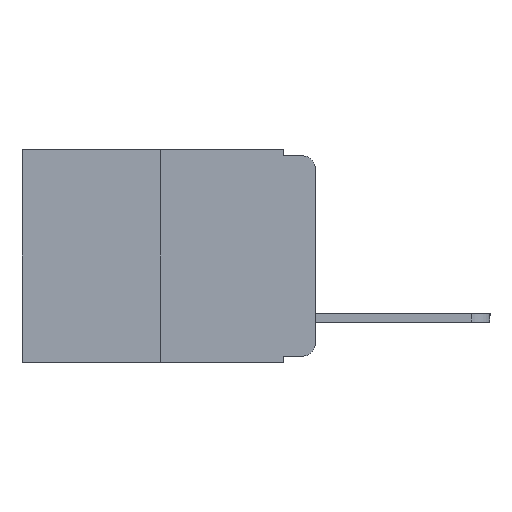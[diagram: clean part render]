
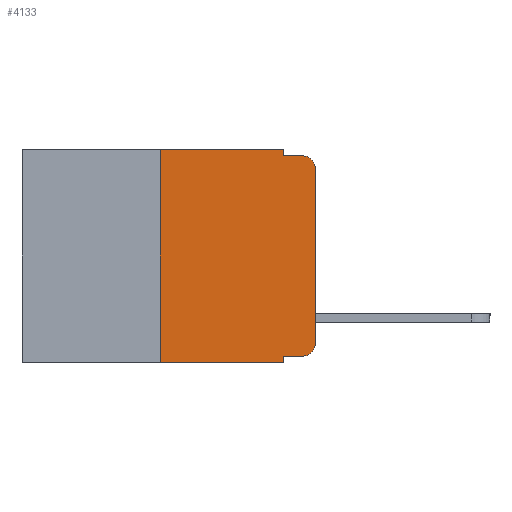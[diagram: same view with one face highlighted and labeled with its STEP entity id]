
A CAD part, left-side view. The second image highlights one B-rep face of the part: STEP entity #4133.
In plain terms, the highlighted planar face has unit normal (-1, 0, 0).
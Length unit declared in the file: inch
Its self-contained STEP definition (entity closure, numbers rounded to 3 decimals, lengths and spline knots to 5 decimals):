
#95 = VERTEX_POINT ( 'NONE', #16208 ) ;
#182 = VERTEX_POINT ( 'NONE', #3348 ) ;
#310 = VECTOR ( 'NONE', #2990, 39.37008 ) ;
#672 = EDGE_CURVE ( 'NONE', #12954, #3378, #6587, .T. ) ;
#984 = ORIENTED_EDGE ( 'NONE', *, *, #6790, .F. ) ;
#1202 = CARTESIAN_POINT ( 'NONE',  ( 0., 0.02, -0.03 ) ) ;
#1562 = CARTESIAN_POINT ( 'NONE',  ( 0., 0.051, 0. ) ) ;
#1575 = VERTEX_POINT ( 'NONE', #4883 ) ;
#1704 = CIRCLE ( 'NONE', #12502, 0.02 ) ;
#2107 = CARTESIAN_POINT ( 'NONE',  ( 0., 0.473, 0. ) ) ;
#2113 = CARTESIAN_POINT ( 'NONE',  ( 0., 0.051, -0.01 ) ) ;
#2175 = ORIENTED_EDGE ( 'NONE', *, *, #2684, .F. ) ;
#2372 = CARTESIAN_POINT ( 'NONE',  ( 0., 0., 0. ) ) ;
#2684 = EDGE_CURVE ( 'NONE', #12954, #6136, #8379, .T. ) ;
#2698 = DIRECTION ( 'NONE',  ( 0., 0., -1. ) ) ;
#2830 = DIRECTION ( 'NONE',  ( 0., 0., 1. ) ) ;
#2990 = DIRECTION ( 'NONE',  ( 0., 0., -1. ) ) ;
#3138 = CARTESIAN_POINT ( 'NONE',  ( 0., 0.051, -0.01 ) ) ;
#3348 = CARTESIAN_POINT ( 'NONE',  ( 0., 0.051, 0. ) ) ;
#3378 = VERTEX_POINT ( 'NONE', #7827 ) ;
#3686 = EDGE_CURVE ( 'NONE', #14609, #1575, #9997, .T. ) ;
#3984 = CARTESIAN_POINT ( 'NONE',  ( 0., 0.051, -0.343 ) ) ;
#4133 = ADVANCED_FACE ( 'NONE', ( #13971 ), #8501, .F. ) ;
#4368 = DIRECTION ( 'NONE',  ( 0., -1., 0. ) ) ;
#4509 = ORIENTED_EDGE ( 'NONE', *, *, #8810, .F. ) ;
#4762 = VECTOR ( 'NONE', #4368, 39.37008 ) ;
#4883 = CARTESIAN_POINT ( 'NONE',  ( 0., 0.25, 0. ) ) ;
#4994 = ORIENTED_EDGE ( 'NONE', *, *, #7572, .F. ) ;
#5941 = VECTOR ( 'NONE', #6303, 39.37008 ) ;
#6136 = VERTEX_POINT ( 'NONE', #3984 ) ;
#6303 = DIRECTION ( 'NONE',  ( 0., -1., 0. ) ) ;
#6587 = LINE ( 'NONE', #9152, #17464 ) ;
#6790 = EDGE_CURVE ( 'NONE', #182, #10097, #16294, .T. ) ;
#7131 = CARTESIAN_POINT ( 'NONE',  ( 0., 0.02, -0.313 ) ) ;
#7145 = DIRECTION ( 'NONE',  ( 0., 0., -1. ) ) ;
#7469 = CARTESIAN_POINT ( 'NONE',  ( 0., 0.02, -0.01 ) ) ;
#7572 = EDGE_CURVE ( 'NONE', #1575, #182, #10010, .T. ) ;
#7827 = CARTESIAN_POINT ( 'NONE',  ( 0., 0.02, -0.333 ) ) ;
#7871 = ORIENTED_EDGE ( 'NONE', *, *, #17929, .T. ) ;
#8071 = DIRECTION ( 'NONE',  ( 0., -1., 0. ) ) ;
#8379 = LINE ( 'NONE', #1562, #310 ) ;
#8501 = PLANE ( 'NONE',  #11015 ) ;
#8629 = DIRECTION ( 'NONE',  ( 0., 0., -1. ) ) ;
#8731 = CARTESIAN_POINT ( 'NONE',  ( 0., 0.25, -0.343 ) ) ;
#8810 = EDGE_CURVE ( 'NONE', #10097, #15462, #9481, .T. ) ;
#9152 = CARTESIAN_POINT ( 'NONE',  ( 0., 0.051, -0.333 ) ) ;
#9210 = DIRECTION ( 'NONE',  ( 0., -1., 0. ) ) ;
#9481 = LINE ( 'NONE', #3138, #5941 ) ;
#9832 = EDGE_CURVE ( 'NONE', #95, #15462, #18821, .T. ) ;
#9986 = ORIENTED_EDGE ( 'NONE', *, *, #672, .T. ) ;
#9997 = LINE ( 'NONE', #13420, #13989 ) ;
#10010 = LINE ( 'NONE', #13739, #16916 ) ;
#10097 = VERTEX_POINT ( 'NONE', #2113 ) ;
#10467 = ORIENTED_EDGE ( 'NONE', *, *, #18996, .T. ) ;
#10726 = ORIENTED_EDGE ( 'NONE', *, *, #10859, .T. ) ;
#10859 = EDGE_CURVE ( 'NONE', #17457, #95, #12681, .T. ) ;
#11015 = AXIS2_PLACEMENT_3D ( 'NONE', #2107, #11992, #16215 ) ;
#11409 = EDGE_LOOP ( 'NONE', ( #10726, #15564, #4509, #984, #4994, #18686, #7871, #2175, #9986, #10467 ) ) ;
#11803 = DIRECTION ( 'NONE',  ( -1., 0., 0. ) ) ;
#11992 = DIRECTION ( 'NONE',  ( 1., 0., 0. ) ) ;
#12053 = CARTESIAN_POINT ( 'NONE',  ( 0., 0., -0.313 ) ) ;
#12390 = CARTESIAN_POINT ( 'NONE',  ( 0., 0.051, -0.333 ) ) ;
#12502 = AXIS2_PLACEMENT_3D ( 'NONE', #7131, #17458, #8629 ) ;
#12681 = LINE ( 'NONE', #2372, #16564 ) ;
#12954 = VERTEX_POINT ( 'NONE', #12390 ) ;
#13420 = CARTESIAN_POINT ( 'NONE',  ( 0., 0.25, 0. ) ) ;
#13739 = CARTESIAN_POINT ( 'NONE',  ( 0., 0.473, 0. ) ) ;
#13971 = FACE_OUTER_BOUND ( 'NONE', #11409, .T. ) ;
#13989 = VECTOR ( 'NONE', #2830, 39.37008 ) ;
#14317 = AXIS2_PLACEMENT_3D ( 'NONE', #1202, #11803, #2698 ) ;
#14609 = VERTEX_POINT ( 'NONE', #8731 ) ;
#14930 = CARTESIAN_POINT ( 'NONE',  ( 0., 0.473, -0.343 ) ) ;
#15462 = VERTEX_POINT ( 'NONE', #7469 ) ;
#15564 = ORIENTED_EDGE ( 'NONE', *, *, #9832, .T. ) ;
#16053 = CARTESIAN_POINT ( 'NONE',  ( 0., 0.051, 0. ) ) ;
#16208 = CARTESIAN_POINT ( 'NONE',  ( 0., 0., -0.03 ) ) ;
#16215 = DIRECTION ( 'NONE',  ( 0., 0., -1. ) ) ;
#16258 = LINE ( 'NONE', #14930, #4762 ) ;
#16294 = LINE ( 'NONE', #16053, #16740 ) ;
#16564 = VECTOR ( 'NONE', #17266, 39.37008 ) ;
#16740 = VECTOR ( 'NONE', #7145, 39.37008 ) ;
#16916 = VECTOR ( 'NONE', #9210, 39.37008 ) ;
#17266 = DIRECTION ( 'NONE',  ( 0., 0., 1. ) ) ;
#17457 = VERTEX_POINT ( 'NONE', #12053 ) ;
#17458 = DIRECTION ( 'NONE',  ( -1., 0., 0. ) ) ;
#17464 = VECTOR ( 'NONE', #8071, 39.37008 ) ;
#17929 = EDGE_CURVE ( 'NONE', #14609, #6136, #16258, .T. ) ;
#18686 = ORIENTED_EDGE ( 'NONE', *, *, #3686, .F. ) ;
#18821 = CIRCLE ( 'NONE', #14317, 0.02 ) ;
#18996 = EDGE_CURVE ( 'NONE', #3378, #17457, #1704, .T. ) ;
